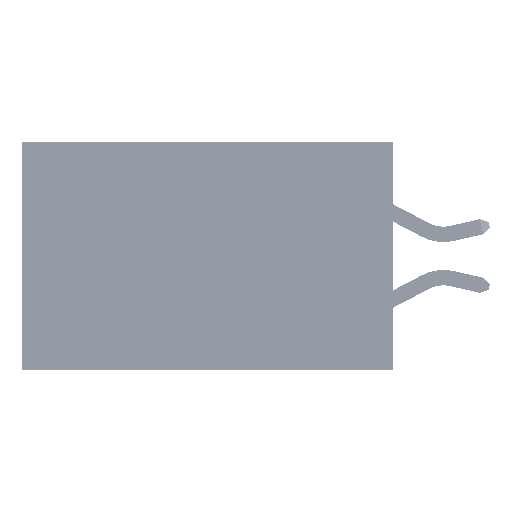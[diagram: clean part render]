
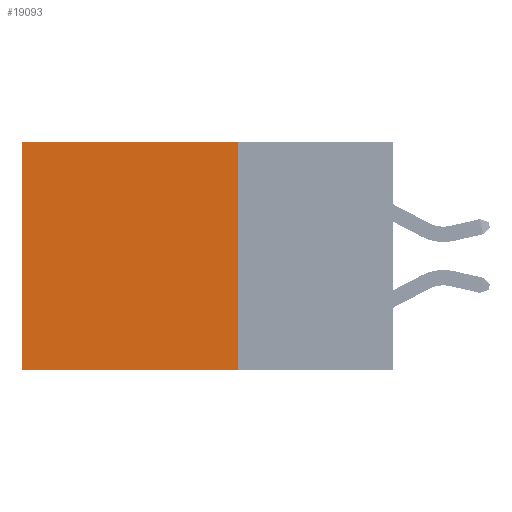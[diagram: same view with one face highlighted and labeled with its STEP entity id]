
A CAD part, left-side view. The second image highlights one B-rep face of the part: STEP entity #19093.
In plain terms, the highlighted planar face has unit normal (-1, 0, 0).
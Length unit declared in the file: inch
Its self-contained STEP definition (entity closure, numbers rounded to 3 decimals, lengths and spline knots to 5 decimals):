
#1347 = AXIS2_PLACEMENT_3D ( 'NONE', #45248, #20489, #8377 ) ;
#7147 = CARTESIAN_POINT ( 'NONE',  ( 0.2875, 0.25, -0.37 ) ) ;
#8128 = EDGE_LOOP ( 'NONE', ( #24832, #19464, #44260, #13817 ) ) ;
#8377 = DIRECTION ( 'NONE',  ( 0., 0., -1. ) ) ;
#8652 = CARTESIAN_POINT ( 'NONE',  ( 0.2875, 0.6, 0. ) ) ;
#10514 = CARTESIAN_POINT ( 'NONE',  ( 0.2875, 0.6, -0.37 ) ) ;
#11870 = VECTOR ( 'NONE', #49879, 39.37008 ) ;
#12534 = VERTEX_POINT ( 'NONE', #10514 ) ;
#13817 = ORIENTED_EDGE ( 'NONE', *, *, #23319, .T. ) ;
#16184 = PLANE ( 'NONE',  #1347 ) ;
#18021 = VERTEX_POINT ( 'NONE', #19565 ) ;
#19093 = ADVANCED_FACE ( 'NONE', ( #49027 ), #16184, .F. ) ;
#19464 = ORIENTED_EDGE ( 'NONE', *, *, #23207, .F. ) ;
#19565 = CARTESIAN_POINT ( 'NONE',  ( 0.2875, 0.25, -0.37 ) ) ;
#20154 = DIRECTION ( 'NONE',  ( 0., 0., -1. ) ) ;
#20489 = DIRECTION ( 'NONE',  ( 1., 0., 0. ) ) ;
#20549 = CARTESIAN_POINT ( 'NONE',  ( 0.2875, 0.25, 0. ) ) ;
#22233 = EDGE_CURVE ( 'NONE', #50513, #18021, #52461, .T. ) ;
#23207 = EDGE_CURVE ( 'NONE', #18021, #12534, #43995, .T. ) ;
#23319 = EDGE_CURVE ( 'NONE', #50513, #25131, #37501, .T. ) ;
#23543 = DIRECTION ( 'NONE',  ( 0., 1., 0. ) ) ;
#24813 = DIRECTION ( 'NONE',  ( 0., 0., -1. ) ) ;
#24832 = ORIENTED_EDGE ( 'NONE', *, *, #50329, .T. ) ;
#25131 = VERTEX_POINT ( 'NONE', #8652 ) ;
#26423 = VECTOR ( 'NONE', #23543, 39.37008 ) ;
#26947 = CARTESIAN_POINT ( 'NONE',  ( 0.2875, 0.25, 0. ) ) ;
#29913 = CARTESIAN_POINT ( 'NONE',  ( 0.2875, 0.6, 0. ) ) ;
#32262 = CARTESIAN_POINT ( 'NONE',  ( 0.2875, 0.25, 0. ) ) ;
#37501 = LINE ( 'NONE', #20549, #11870 ) ;
#41870 = VECTOR ( 'NONE', #20154, 39.37008 ) ;
#43995 = LINE ( 'NONE', #7147, #26423 ) ;
#44260 = ORIENTED_EDGE ( 'NONE', *, *, #22233, .F. ) ;
#45248 = CARTESIAN_POINT ( 'NONE',  ( 0.2875, 0.25, 0. ) ) ;
#49027 = FACE_OUTER_BOUND ( 'NONE', #8128, .T. ) ;
#49879 = DIRECTION ( 'NONE',  ( 0., 1., 0. ) ) ;
#50329 = EDGE_CURVE ( 'NONE', #25131, #12534, #50381, .T. ) ;
#50381 = LINE ( 'NONE', #29913, #52040 ) ;
#50513 = VERTEX_POINT ( 'NONE', #26947 ) ;
#52040 = VECTOR ( 'NONE', #24813, 39.37008 ) ;
#52461 = LINE ( 'NONE', #32262, #41870 ) ;
